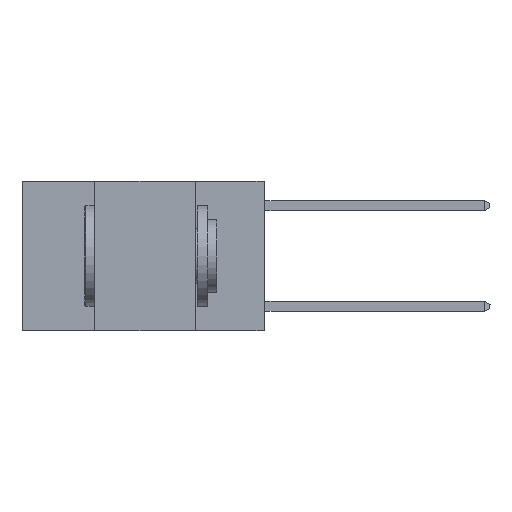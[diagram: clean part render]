
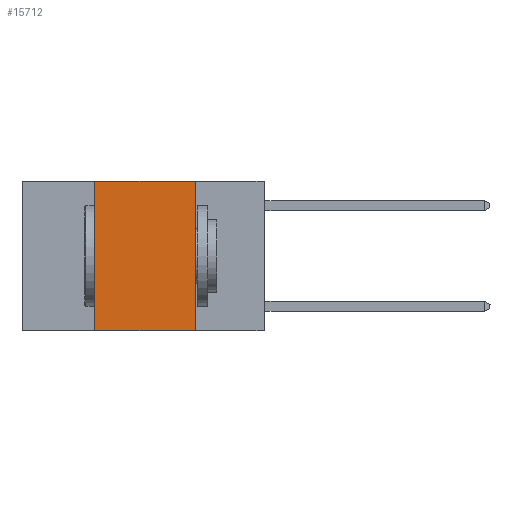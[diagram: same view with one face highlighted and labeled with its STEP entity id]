
A CAD part, left-side view. The second image highlights one B-rep face of the part: STEP entity #15712.
In plain terms, the highlighted planar face has unit normal (-1, 0, 0).
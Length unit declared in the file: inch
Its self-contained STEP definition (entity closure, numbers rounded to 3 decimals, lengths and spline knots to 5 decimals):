
#430 = VECTOR ( 'NONE', #655, 39.37008 ) ;
#655 = DIRECTION ( 'NONE',  ( 0., -1., 0. ) ) ;
#940 = LINE ( 'NONE', #3200, #16348 ) ;
#1052 = ORIENTED_EDGE ( 'NONE', *, *, #10568, .T. ) ;
#1726 = EDGE_CURVE ( 'NONE', #1891, #3267, #940, .T. ) ;
#1891 = VERTEX_POINT ( 'NONE', #2915 ) ;
#1955 = DIRECTION ( 'NONE',  ( 0., 0., 1. ) ) ;
#2338 = CARTESIAN_POINT ( 'NONE',  ( 0., 0.17, 0. ) ) ;
#2481 = CARTESIAN_POINT ( 'NONE',  ( 0., 0.17, -0.37 ) ) ;
#2915 = CARTESIAN_POINT ( 'NONE',  ( 0., 0.42, -0.37 ) ) ;
#3007 = FACE_OUTER_BOUND ( 'NONE', #15433, .T. ) ;
#3200 = CARTESIAN_POINT ( 'NONE',  ( 0., 0.42, 0. ) ) ;
#3267 = VERTEX_POINT ( 'NONE', #12271 ) ;
#3778 = CARTESIAN_POINT ( 'NONE',  ( 0., 0.6, 0. ) ) ;
#4618 = AXIS2_PLACEMENT_3D ( 'NONE', #3778, #14876, #5325 ) ;
#5254 = LINE ( 'NONE', #2338, #14203 ) ;
#5325 = DIRECTION ( 'NONE',  ( 0., 0., -1. ) ) ;
#6121 = DIRECTION ( 'NONE',  ( 0., -1., 0. ) ) ;
#6880 = EDGE_CURVE ( 'NONE', #3267, #19314, #8606, .T. ) ;
#8006 = ORIENTED_EDGE ( 'NONE', *, *, #1726, .F. ) ;
#8122 = VECTOR ( 'NONE', #6121, 39.37008 ) ;
#8201 = ORIENTED_EDGE ( 'NONE', *, *, #6880, .F. ) ;
#8606 = LINE ( 'NONE', #17264, #8122 ) ;
#8616 = DIRECTION ( 'NONE',  ( 0., 0., -1. ) ) ;
#9148 = EDGE_CURVE ( 'NONE', #19314, #11292, #5254, .T. ) ;
#10568 = EDGE_CURVE ( 'NONE', #1891, #11292, #17320, .T. ) ;
#11292 = VERTEX_POINT ( 'NONE', #2481 ) ;
#12271 = CARTESIAN_POINT ( 'NONE',  ( 0., 0.42, 0. ) ) ;
#13302 = CARTESIAN_POINT ( 'NONE',  ( 0., 0.6, -0.37 ) ) ;
#14203 = VECTOR ( 'NONE', #8616, 39.37008 ) ;
#14876 = DIRECTION ( 'NONE',  ( 1., 0., 0. ) ) ;
#15029 = ORIENTED_EDGE ( 'NONE', *, *, #9148, .F. ) ;
#15433 = EDGE_LOOP ( 'NONE', ( #15029, #8201, #8006, #1052 ) ) ;
#15712 = ADVANCED_FACE ( 'NONE', ( #3007 ), #16427, .F. ) ;
#16348 = VECTOR ( 'NONE', #1955, 39.37008 ) ;
#16427 = PLANE ( 'NONE',  #4618 ) ;
#17264 = CARTESIAN_POINT ( 'NONE',  ( 0., 0.6, 0. ) ) ;
#17320 = LINE ( 'NONE', #13302, #430 ) ;
#18327 = CARTESIAN_POINT ( 'NONE',  ( 0., 0.17, 0. ) ) ;
#19314 = VERTEX_POINT ( 'NONE', #18327 ) ;
